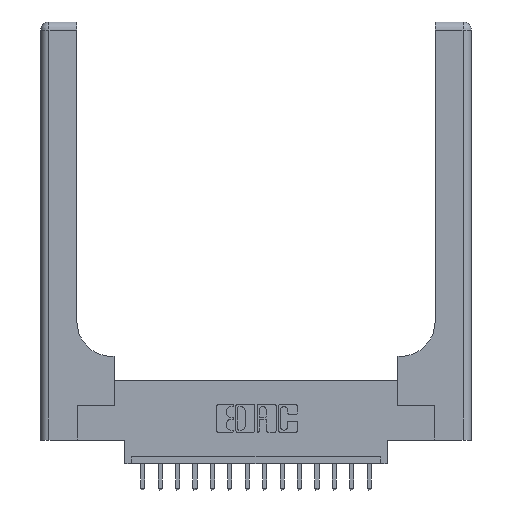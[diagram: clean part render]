
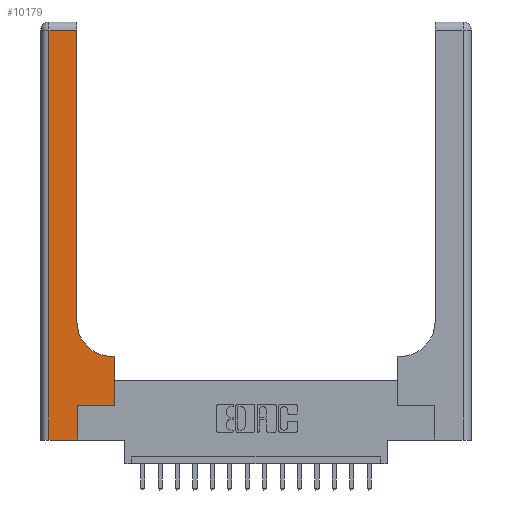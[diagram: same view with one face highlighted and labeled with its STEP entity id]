
A CAD part, top view. The second image highlights one B-rep face of the part: STEP entity #10179.
In plain terms, the highlighted planar face has unit normal (0, 0, 1).
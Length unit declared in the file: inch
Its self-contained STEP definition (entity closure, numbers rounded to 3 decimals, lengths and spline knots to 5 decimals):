
#26 = EDGE_CURVE ( 'NONE', #8439, #2645, #7109, .T. ) ;
#284 = CARTESIAN_POINT ( 'NONE',  ( 0.06, 0., 0.37 ) ) ;
#500 = EDGE_CURVE ( 'NONE', #8001, #11749, #7320, .T. ) ;
#705 = CARTESIAN_POINT ( 'NONE',  ( 0., 0., 0.37 ) ) ;
#980 = CARTESIAN_POINT ( 'NONE',  ( 0.51, 0.6, 0.37 ) ) ;
#1115 = CARTESIAN_POINT ( 'NONE',  ( 0., 3., 0.37 ) ) ;
#1473 = CARTESIAN_POINT ( 'NONE',  ( 0.26, 2.94, 0.37 ) ) ;
#1743 = DIRECTION ( 'NONE',  ( -1., 0., 0. ) ) ;
#2032 = VECTOR ( 'NONE', #10393, 39.37008 ) ;
#2645 = VERTEX_POINT ( 'NONE', #15380 ) ;
#2876 = FACE_OUTER_BOUND ( 'NONE', #14728, .T. ) ;
#2951 = EDGE_CURVE ( 'NONE', #15314, #8439, #6376, .T. ) ;
#3251 = CARTESIAN_POINT ( 'NONE',  ( 0.26, 0.6, 0.37 ) ) ;
#3257 = VERTEX_POINT ( 'NONE', #5741 ) ;
#3497 = DIRECTION ( 'NONE',  ( 0., -1., 0. ) ) ;
#3799 = CARTESIAN_POINT ( 'NONE',  ( 0., 2.94, 0.37 ) ) ;
#3868 = EDGE_CURVE ( 'NONE', #5566, #15314, #3968, .T. ) ;
#3927 = DIRECTION ( 'NONE',  ( 0., 0., -1. ) ) ;
#3962 = LINE ( 'NONE', #3251, #12563 ) ;
#3968 = LINE ( 'NONE', #10502, #2032 ) ;
#4523 = CARTESIAN_POINT ( 'NONE',  ( 0.528, 0.25, 0.37 ) ) ;
#4639 = DIRECTION ( 'NONE',  ( 0., 1., 0. ) ) ;
#4812 = LINE ( 'NONE', #705, #10595 ) ;
#5118 = EDGE_CURVE ( 'NONE', #11749, #11803, #11411, .T. ) ;
#5249 = DIRECTION ( 'NONE',  ( 0., 0., -1. ) ) ;
#5320 = CARTESIAN_POINT ( 'NONE',  ( 0.265, 0., 0.37 ) ) ;
#5394 = ORIENTED_EDGE ( 'NONE', *, *, #13177, .T. ) ;
#5566 = VERTEX_POINT ( 'NONE', #5320 ) ;
#5667 = VERTEX_POINT ( 'NONE', #284 ) ;
#5741 = CARTESIAN_POINT ( 'NONE',  ( 0.06, 2.94, 0.37 ) ) ;
#6376 = LINE ( 'NONE', #13638, #8949 ) ;
#6699 = ORIENTED_EDGE ( 'NONE', *, *, #11310, .T. ) ;
#7109 = LINE ( 'NONE', #14301, #17671 ) ;
#7203 = CARTESIAN_POINT ( 'NONE',  ( 0.06, 3., 0.37 ) ) ;
#7320 = CIRCLE ( 'NONE', #14148, 0.25 ) ;
#7924 = ORIENTED_EDGE ( 'NONE', *, *, #2951, .T. ) ;
#8001 = VERTEX_POINT ( 'NONE', #980 ) ;
#8173 = CARTESIAN_POINT ( 'NONE',  ( 0.26, 3., 0.37 ) ) ;
#8369 = ORIENTED_EDGE ( 'NONE', *, *, #26, .T. ) ;
#8419 = VECTOR ( 'NONE', #10984, 39.37008 ) ;
#8439 = VERTEX_POINT ( 'NONE', #4523 ) ;
#8501 = VECTOR ( 'NONE', #3497, 39.37008 ) ;
#8839 = VECTOR ( 'NONE', #10593, 39.37008 ) ;
#8949 = VECTOR ( 'NONE', #9799, 39.37008 ) ;
#9799 = DIRECTION ( 'NONE',  ( 1., 0., 0. ) ) ;
#10179 = ADVANCED_FACE ( 'NONE', ( #2876 ), #10813, .F. ) ;
#10208 = DIRECTION ( 'NONE',  ( 1., 0., 0. ) ) ;
#10332 = AXIS2_PLACEMENT_3D ( 'NONE', #1115, #5249, #10872 ) ;
#10393 = DIRECTION ( 'NONE',  ( 0., 1., 0. ) ) ;
#10502 = CARTESIAN_POINT ( 'NONE',  ( 0.265, 0., 0.37 ) ) ;
#10593 = DIRECTION ( 'NONE',  ( -1., 0., 0. ) ) ;
#10595 = VECTOR ( 'NONE', #10208, 39.37008 ) ;
#10813 = PLANE ( 'NONE',  #10332 ) ;
#10872 = DIRECTION ( 'NONE',  ( -1., 0., 0. ) ) ;
#10984 = DIRECTION ( 'NONE',  ( 0., 1., 0. ) ) ;
#11077 = CARTESIAN_POINT ( 'NONE',  ( 0.51, 0.85, 0.37 ) ) ;
#11204 = EDGE_CURVE ( 'NONE', #2645, #8001, #3962, .T. ) ;
#11237 = ORIENTED_EDGE ( 'NONE', *, *, #5118, .T. ) ;
#11310 = EDGE_CURVE ( 'NONE', #3257, #5667, #16215, .T. ) ;
#11409 = LINE ( 'NONE', #3799, #8839 ) ;
#11411 = LINE ( 'NONE', #8173, #8419 ) ;
#11749 = VERTEX_POINT ( 'NONE', #16586 ) ;
#11803 = VERTEX_POINT ( 'NONE', #1473 ) ;
#12278 = EDGE_CURVE ( 'NONE', #5667, #5566, #4812, .T. ) ;
#12563 = VECTOR ( 'NONE', #1743, 39.37008 ) ;
#12960 = ORIENTED_EDGE ( 'NONE', *, *, #12278, .T. ) ;
#13177 = EDGE_CURVE ( 'NONE', #11803, #3257, #11409, .T. ) ;
#13546 = DIRECTION ( 'NONE',  ( 1., 0., 0. ) ) ;
#13613 = ORIENTED_EDGE ( 'NONE', *, *, #500, .T. ) ;
#13638 = CARTESIAN_POINT ( 'NONE',  ( 0.265, 0.25, 0.37 ) ) ;
#14148 = AXIS2_PLACEMENT_3D ( 'NONE', #11077, #3927, #13546 ) ;
#14301 = CARTESIAN_POINT ( 'NONE',  ( 0.528, 0.25, 0.37 ) ) ;
#14728 = EDGE_LOOP ( 'NONE', ( #11237, #5394, #6699, #12960, #16374, #7924, #8369, #15851, #13613 ) ) ;
#14865 = CARTESIAN_POINT ( 'NONE',  ( 0.265, 0.25, 0.37 ) ) ;
#15314 = VERTEX_POINT ( 'NONE', #14865 ) ;
#15380 = CARTESIAN_POINT ( 'NONE',  ( 0.528, 0.6, 0.37 ) ) ;
#15851 = ORIENTED_EDGE ( 'NONE', *, *, #11204, .T. ) ;
#16215 = LINE ( 'NONE', #7203, #8501 ) ;
#16374 = ORIENTED_EDGE ( 'NONE', *, *, #3868, .T. ) ;
#16586 = CARTESIAN_POINT ( 'NONE',  ( 0.26, 0.85, 0.37 ) ) ;
#17671 = VECTOR ( 'NONE', #4639, 39.37008 ) ;
